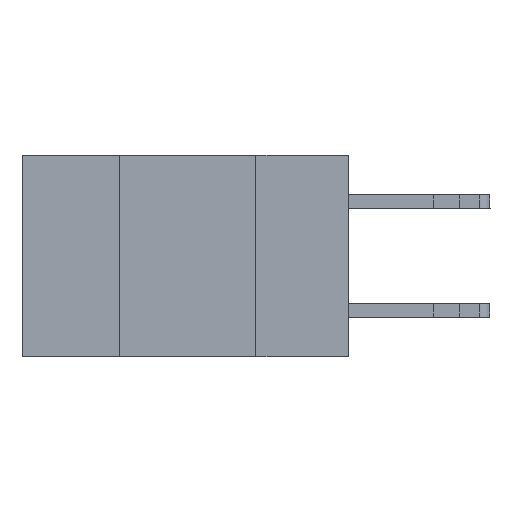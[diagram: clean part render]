
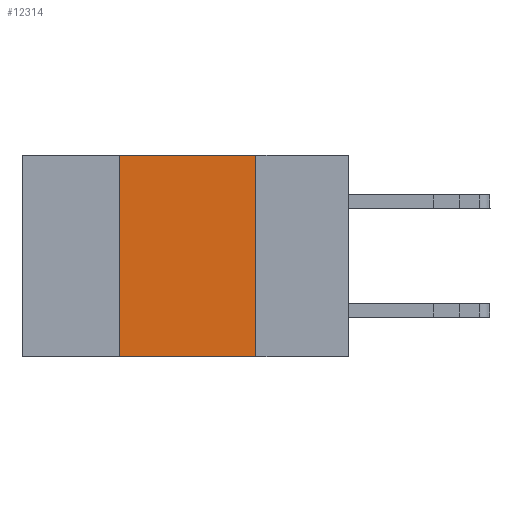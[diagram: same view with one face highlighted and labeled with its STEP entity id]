
A CAD part, left-side view. The second image highlights one B-rep face of the part: STEP entity #12314.
In plain terms, the highlighted planar face has unit normal (-1, 0, 0).
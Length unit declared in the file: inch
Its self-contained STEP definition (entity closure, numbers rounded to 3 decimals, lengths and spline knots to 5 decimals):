
#83 = VECTOR ( 'NONE', #13552, 39.37008 ) ;
#372 = DIRECTION ( 'NONE',  ( 1., 0., 0. ) ) ;
#772 = EDGE_CURVE ( 'NONE', #9869, #8902, #3886, .T. ) ;
#1805 = CARTESIAN_POINT ( 'NONE',  ( 0., 0.17, 0. ) ) ;
#2362 = EDGE_CURVE ( 'NONE', #8902, #10592, #6076, .T. ) ;
#2841 = VECTOR ( 'NONE', #8185, 39.37008 ) ;
#3770 = LINE ( 'NONE', #6917, #2841 ) ;
#3886 = LINE ( 'NONE', #9096, #5012 ) ;
#4464 = CARTESIAN_POINT ( 'NONE',  ( 0., 0.42, 0. ) ) ;
#5012 = VECTOR ( 'NONE', #11364, 39.37008 ) ;
#5627 = FACE_OUTER_BOUND ( 'NONE', #7371, .T. ) ;
#6076 = LINE ( 'NONE', #10404, #11832 ) ;
#6537 = CARTESIAN_POINT ( 'NONE',  ( 0., 0.6, 0. ) ) ;
#6748 = PLANE ( 'NONE',  #8890 ) ;
#6917 = CARTESIAN_POINT ( 'NONE',  ( 0., 0.6, -0.37 ) ) ;
#7371 = EDGE_LOOP ( 'NONE', ( #12523, #8006, #8231, #11351 ) ) ;
#7914 = EDGE_CURVE ( 'NONE', #9509, #9869, #10333, .T. ) ;
#8006 = ORIENTED_EDGE ( 'NONE', *, *, #772, .F. ) ;
#8128 = DIRECTION ( 'NONE',  ( 0., 0., -1. ) ) ;
#8185 = DIRECTION ( 'NONE',  ( 0., -1., 0. ) ) ;
#8231 = ORIENTED_EDGE ( 'NONE', *, *, #7914, .F. ) ;
#8890 = AXIS2_PLACEMENT_3D ( 'NONE', #6537, #372, #10868 ) ;
#8902 = VERTEX_POINT ( 'NONE', #1805 ) ;
#9096 = CARTESIAN_POINT ( 'NONE',  ( 0., 0.6, 0. ) ) ;
#9267 = CARTESIAN_POINT ( 'NONE',  ( 0., 0.42, -0.37 ) ) ;
#9509 = VERTEX_POINT ( 'NONE', #12230 ) ;
#9869 = VERTEX_POINT ( 'NONE', #4464 ) ;
#10333 = LINE ( 'NONE', #9267, #83 ) ;
#10404 = CARTESIAN_POINT ( 'NONE',  ( 0., 0.17, -0.37 ) ) ;
#10592 = VERTEX_POINT ( 'NONE', #11496 ) ;
#10868 = DIRECTION ( 'NONE',  ( 0., 0., -1. ) ) ;
#11351 = ORIENTED_EDGE ( 'NONE', *, *, #11884, .T. ) ;
#11364 = DIRECTION ( 'NONE',  ( 0., -1., 0. ) ) ;
#11496 = CARTESIAN_POINT ( 'NONE',  ( 0., 0.17, -0.37 ) ) ;
#11832 = VECTOR ( 'NONE', #8128, 39.37008 ) ;
#11884 = EDGE_CURVE ( 'NONE', #9509, #10592, #3770, .T. ) ;
#12230 = CARTESIAN_POINT ( 'NONE',  ( 0., 0.42, -0.37 ) ) ;
#12314 = ADVANCED_FACE ( 'NONE', ( #5627 ), #6748, .F. ) ;
#12523 = ORIENTED_EDGE ( 'NONE', *, *, #2362, .F. ) ;
#13552 = DIRECTION ( 'NONE',  ( 0., 0., 1. ) ) ;
